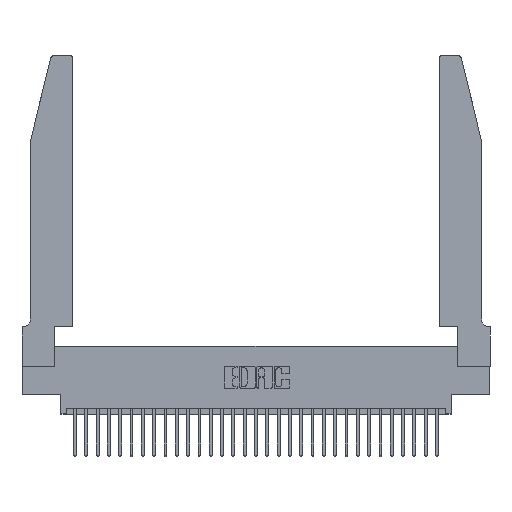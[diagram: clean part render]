
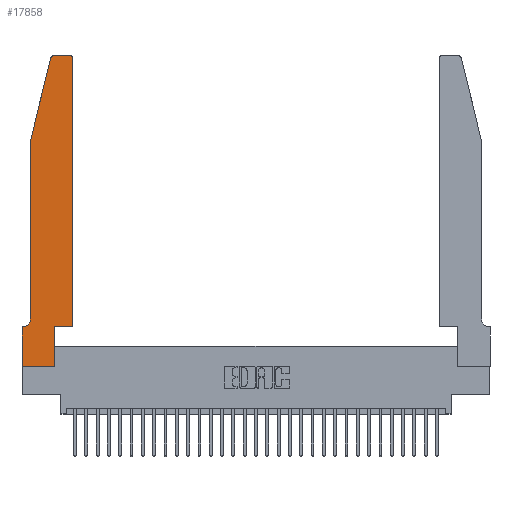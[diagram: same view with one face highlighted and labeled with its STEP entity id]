
A CAD part, top view. The second image highlights one B-rep face of the part: STEP entity #17858.
In plain terms, the highlighted planar face has unit normal (0, 0, 1).
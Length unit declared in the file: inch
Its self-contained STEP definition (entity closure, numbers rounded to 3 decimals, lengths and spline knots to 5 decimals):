
#91 = ORIENTED_EDGE ( 'NONE', *, *, #32002, .T. ) ;
#289 = DIRECTION ( 'NONE',  ( 0., -1., 0. ) ) ;
#931 = LINE ( 'NONE', #9521, #12707 ) ;
#1112 = DIRECTION ( 'NONE',  ( 1., 0., 0. ) ) ;
#1977 = ORIENTED_EDGE ( 'NONE', *, *, #8854, .T. ) ;
#2219 = DIRECTION ( 'NONE',  ( 1., 0., 0. ) ) ;
#2454 = EDGE_CURVE ( 'NONE', #11379, #5293, #4017, .T. ) ;
#2731 = VECTOR ( 'NONE', #9300, 39.37008 ) ;
#2996 = VECTOR ( 'NONE', #17636, 39.37008 ) ;
#3240 = CIRCLE ( 'NONE', #31952, 0.03 ) ;
#3850 = VERTEX_POINT ( 'NONE', #12684 ) ;
#4017 = LINE ( 'NONE', #16629, #23124 ) ;
#4131 = ORIENTED_EDGE ( 'NONE', *, *, #24636, .T. ) ;
#4196 = VECTOR ( 'NONE', #21662, 39.37008 ) ;
#4248 = EDGE_CURVE ( 'NONE', #4612, #19588, #27574, .T. ) ;
#4431 = DIRECTION ( 'NONE',  ( 0., 0., -1. ) ) ;
#4612 = VERTEX_POINT ( 'NONE', #28372 ) ;
#5238 = CARTESIAN_POINT ( 'NONE',  ( 0.2865, 0., 0.37 ) ) ;
#5293 = VERTEX_POINT ( 'NONE', #16439 ) ;
#5594 = CIRCLE ( 'NONE', #6543, 0.03 ) ;
#5885 = CARTESIAN_POINT ( 'NONE',  ( 0.25487, 2.72718, 0.37 ) ) ;
#6543 = AXIS2_PLACEMENT_3D ( 'NONE', #30755, #16141, #1112 ) ;
#6629 = VERTEX_POINT ( 'NONE', #31039 ) ;
#6783 = CARTESIAN_POINT ( 'NONE',  ( 0.4505, 0.35, 0.37 ) ) ;
#7004 = DIRECTION ( 'NONE',  ( 0., -1., 0. ) ) ;
#8234 = VERTEX_POINT ( 'NONE', #10662 ) ;
#8854 = EDGE_CURVE ( 'NONE', #3850, #15867, #18313, .T. ) ;
#9116 = CARTESIAN_POINT ( 'NONE',  ( 0., 0., 0.37 ) ) ;
#9300 = DIRECTION ( 'NONE',  ( 1., 0., 0. ) ) ;
#9521 = CARTESIAN_POINT ( 'NONE',  ( 0.0755, 2., 0.37 ) ) ;
#9781 = EDGE_CURVE ( 'NONE', #16200, #4612, #17499, .T. ) ;
#10002 = DIRECTION ( 'NONE',  ( 0., 0., 1. ) ) ;
#10492 = LINE ( 'NONE', #12627, #2996 ) ;
#10628 = EDGE_CURVE ( 'NONE', #8234, #11535, #19754, .T. ) ;
#10662 = CARTESIAN_POINT ( 'NONE',  ( 0.0755, 0.42, 0.37 ) ) ;
#11375 = ORIENTED_EDGE ( 'NONE', *, *, #2454, .T. ) ;
#11379 = VERTEX_POINT ( 'NONE', #12712 ) ;
#11535 = VERTEX_POINT ( 'NONE', #30406 ) ;
#11551 = ORIENTED_EDGE ( 'NONE', *, *, #4248, .T. ) ;
#12195 = PLANE ( 'NONE',  #29939 ) ;
#12269 = CARTESIAN_POINT ( 'NONE',  ( 0.4505, 2.72, 0.37 ) ) ;
#12503 = ORIENTED_EDGE ( 'NONE', *, *, #28154, .T. ) ;
#12627 = CARTESIAN_POINT ( 'NONE',  ( 0., 0., 0.37 ) ) ;
#12684 = CARTESIAN_POINT ( 'NONE',  ( 0., 0.35, 0.37 ) ) ;
#12707 = VECTOR ( 'NONE', #7004, 39.37008 ) ;
#12712 = CARTESIAN_POINT ( 'NONE',  ( 0.4205, 2.75, 0.37 ) ) ;
#12767 = CARTESIAN_POINT ( 'NONE',  ( 0.0755, 2., 0.37 ) ) ;
#13437 = DIRECTION ( 'NONE',  ( 0., 1., 0. ) ) ;
#14713 = CARTESIAN_POINT ( 'NONE',  ( 0., 0.35, 0.37 ) ) ;
#15867 = VERTEX_POINT ( 'NONE', #9116 ) ;
#16141 = DIRECTION ( 'NONE',  ( 0., 0., 1. ) ) ;
#16200 = VERTEX_POINT ( 'NONE', #5238 ) ;
#16439 = CARTESIAN_POINT ( 'NONE',  ( 0.284, 2.75, 0.37 ) ) ;
#16490 = ORIENTED_EDGE ( 'NONE', *, *, #10628, .T. ) ;
#16590 = AXIS2_PLACEMENT_3D ( 'NONE', #19384, #4431, #21879 ) ;
#16629 = CARTESIAN_POINT ( 'NONE',  ( 0.2605, 2.75, 0.37 ) ) ;
#17022 = CARTESIAN_POINT ( 'NONE',  ( 0.4505, 0.35, 0.37 ) ) ;
#17218 = DIRECTION ( 'NONE',  ( 0., 0., 1. ) ) ;
#17433 = CARTESIAN_POINT ( 'NONE',  ( 0.0755, 0.35, 0.37 ) ) ;
#17499 = LINE ( 'NONE', #30609, #24805 ) ;
#17636 = DIRECTION ( 'NONE',  ( 1., 0., 0. ) ) ;
#17858 = ADVANCED_FACE ( 'NONE', ( #29260 ), #12195, .T. ) ;
#18313 = LINE ( 'NONE', #25095, #30537 ) ;
#18562 = EDGE_CURVE ( 'NONE', #20336, #11379, #3240, .T. ) ;
#18634 = LINE ( 'NONE', #17433, #30098 ) ;
#19156 = CARTESIAN_POINT ( 'NONE',  ( 0.4505, 0.35, 0.37 ) ) ;
#19299 = VERTEX_POINT ( 'NONE', #5885 ) ;
#19384 = CARTESIAN_POINT ( 'NONE',  ( 0.0055, 0.42, 0.37 ) ) ;
#19588 = VERTEX_POINT ( 'NONE', #17022 ) ;
#19754 = CIRCLE ( 'NONE', #16590, 0.07 ) ;
#20150 = DIRECTION ( 'NONE',  ( -0.239, -0.971, 0. ) ) ;
#20239 = ORIENTED_EDGE ( 'NONE', *, *, #31963, .T. ) ;
#20336 = VERTEX_POINT ( 'NONE', #12269 ) ;
#21320 = ORIENTED_EDGE ( 'NONE', *, *, #21850, .T. ) ;
#21662 = DIRECTION ( 'NONE',  ( 0., 1., 0. ) ) ;
#21850 = EDGE_CURVE ( 'NONE', #19299, #6629, #22610, .T. ) ;
#21879 = DIRECTION ( 'NONE',  ( -1., 0., 0. ) ) ;
#22610 = LINE ( 'NONE', #12767, #27542 ) ;
#23124 = VECTOR ( 'NONE', #26387, 39.37008 ) ;
#24041 = LINE ( 'NONE', #19156, #4196 ) ;
#24636 = EDGE_CURVE ( 'NONE', #6629, #8234, #931, .T. ) ;
#24805 = VECTOR ( 'NONE', #13437, 39.37008 ) ;
#24807 = CARTESIAN_POINT ( 'NONE',  ( 0.4205, 2.72, 0.37 ) ) ;
#25095 = CARTESIAN_POINT ( 'NONE',  ( 0., 0., 0.37 ) ) ;
#26387 = DIRECTION ( 'NONE',  ( -1., 0., 0. ) ) ;
#26515 = ORIENTED_EDGE ( 'NONE', *, *, #9781, .T. ) ;
#27247 = DIRECTION ( 'NONE',  ( 1., 0., 0. ) ) ;
#27542 = VECTOR ( 'NONE', #20150, 39.37008 ) ;
#27574 = LINE ( 'NONE', #6783, #2731 ) ;
#28154 = EDGE_CURVE ( 'NONE', #5293, #19299, #5594, .T. ) ;
#28372 = CARTESIAN_POINT ( 'NONE',  ( 0.2865, 0.35, 0.37 ) ) ;
#29042 = ORIENTED_EDGE ( 'NONE', *, *, #31777, .T. ) ;
#29260 = FACE_OUTER_BOUND ( 'NONE', #30187, .T. ) ;
#29605 = DIRECTION ( 'NONE',  ( -1., 0., 0. ) ) ;
#29939 = AXIS2_PLACEMENT_3D ( 'NONE', #14713, #17218, #2219 ) ;
#30098 = VECTOR ( 'NONE', #29605, 39.37008 ) ;
#30187 = EDGE_LOOP ( 'NONE', ( #11375, #12503, #21320, #4131, #16490, #20239, #1977, #91, #26515, #11551, #29042, #30759 ) ) ;
#30406 = CARTESIAN_POINT ( 'NONE',  ( 0.0055, 0.35, 0.37 ) ) ;
#30537 = VECTOR ( 'NONE', #289, 39.37008 ) ;
#30609 = CARTESIAN_POINT ( 'NONE',  ( 0.2865, 0.35, 0.37 ) ) ;
#30755 = CARTESIAN_POINT ( 'NONE',  ( 0.284, 2.72, 0.37 ) ) ;
#30759 = ORIENTED_EDGE ( 'NONE', *, *, #18562, .T. ) ;
#31039 = CARTESIAN_POINT ( 'NONE',  ( 0.0755, 2., 0.37 ) ) ;
#31777 = EDGE_CURVE ( 'NONE', #19588, #20336, #24041, .T. ) ;
#31952 = AXIS2_PLACEMENT_3D ( 'NONE', #24807, #10002, #27247 ) ;
#31963 = EDGE_CURVE ( 'NONE', #11535, #3850, #18634, .T. ) ;
#32002 = EDGE_CURVE ( 'NONE', #15867, #16200, #10492, .T. ) ;
